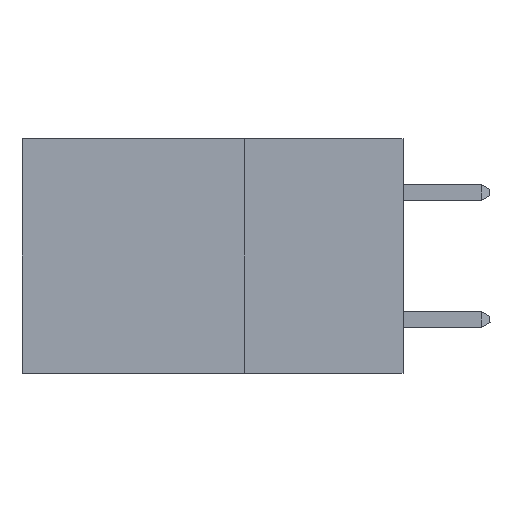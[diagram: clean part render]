
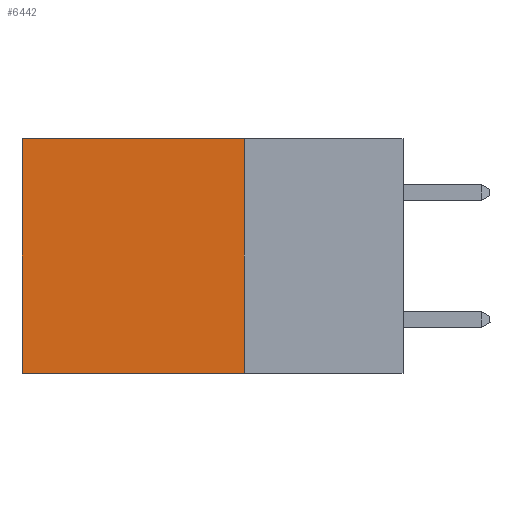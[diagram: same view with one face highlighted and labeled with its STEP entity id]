
A CAD part, left-side view. The second image highlights one B-rep face of the part: STEP entity #6442.
In plain terms, the highlighted planar face has unit normal (-1, 0, 0).
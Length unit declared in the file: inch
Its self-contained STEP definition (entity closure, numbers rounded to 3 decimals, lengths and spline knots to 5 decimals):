
#401 = ORIENTED_EDGE ( 'NONE', *, *, #4273, .T. ) ;
#1437 = DIRECTION ( 'NONE',  ( 0., 0., -1. ) ) ;
#1697 = FACE_OUTER_BOUND ( 'NONE', #1911, .T. ) ;
#1703 = CARTESIAN_POINT ( 'NONE',  ( 0.2875, 0.6, 0. ) ) ;
#1901 = CARTESIAN_POINT ( 'NONE',  ( 0.2875, 0.25, -0.37 ) ) ;
#1911 = EDGE_LOOP ( 'NONE', ( #8111, #12363, #10837, #401 ) ) ;
#2025 = PLANE ( 'NONE',  #9320 ) ;
#2035 = LINE ( 'NONE', #1901, #11198 ) ;
#2527 = LINE ( 'NONE', #5498, #13694 ) ;
#2664 = CARTESIAN_POINT ( 'NONE',  ( 0.2875, 0.6, 0. ) ) ;
#3172 = EDGE_CURVE ( 'NONE', #9579, #8282, #2035, .T. ) ;
#4078 = DIRECTION ( 'NONE',  ( 0., 1., 0. ) ) ;
#4273 = EDGE_CURVE ( 'NONE', #10352, #10081, #10495, .T. ) ;
#4377 = VECTOR ( 'NONE', #4078, 39.37008 ) ;
#4444 = EDGE_CURVE ( 'NONE', #10352, #9579, #2527, .T. ) ;
#4553 = DIRECTION ( 'NONE',  ( 1., 0., 0. ) ) ;
#4574 = CARTESIAN_POINT ( 'NONE',  ( 0.2875, 0.25, -0.37 ) ) ;
#5007 = CARTESIAN_POINT ( 'NONE',  ( 0.2875, 0.25, 0. ) ) ;
#5134 = EDGE_CURVE ( 'NONE', #10081, #8282, #5447, .T. ) ;
#5447 = LINE ( 'NONE', #2664, #13361 ) ;
#5498 = CARTESIAN_POINT ( 'NONE',  ( 0.2875, 0.25, 0. ) ) ;
#6442 = ADVANCED_FACE ( 'NONE', ( #1697 ), #2025, .F. ) ;
#8013 = DIRECTION ( 'NONE',  ( 0., 0., -1. ) ) ;
#8111 = ORIENTED_EDGE ( 'NONE', *, *, #5134, .T. ) ;
#8282 = VERTEX_POINT ( 'NONE', #12185 ) ;
#8509 = DIRECTION ( 'NONE',  ( 0., 1., 0. ) ) ;
#8752 = CARTESIAN_POINT ( 'NONE',  ( 0.2875, 0.25, 0. ) ) ;
#9320 = AXIS2_PLACEMENT_3D ( 'NONE', #8752, #4553, #1437 ) ;
#9579 = VERTEX_POINT ( 'NONE', #4574 ) ;
#10049 = DIRECTION ( 'NONE',  ( 0., 0., -1. ) ) ;
#10081 = VERTEX_POINT ( 'NONE', #1703 ) ;
#10352 = VERTEX_POINT ( 'NONE', #13104 ) ;
#10495 = LINE ( 'NONE', #5007, #4377 ) ;
#10837 = ORIENTED_EDGE ( 'NONE', *, *, #4444, .F. ) ;
#11198 = VECTOR ( 'NONE', #8509, 39.37008 ) ;
#12185 = CARTESIAN_POINT ( 'NONE',  ( 0.2875, 0.6, -0.37 ) ) ;
#12363 = ORIENTED_EDGE ( 'NONE', *, *, #3172, .F. ) ;
#13104 = CARTESIAN_POINT ( 'NONE',  ( 0.2875, 0.25, 0. ) ) ;
#13361 = VECTOR ( 'NONE', #8013, 39.37008 ) ;
#13694 = VECTOR ( 'NONE', #10049, 39.37008 ) ;
